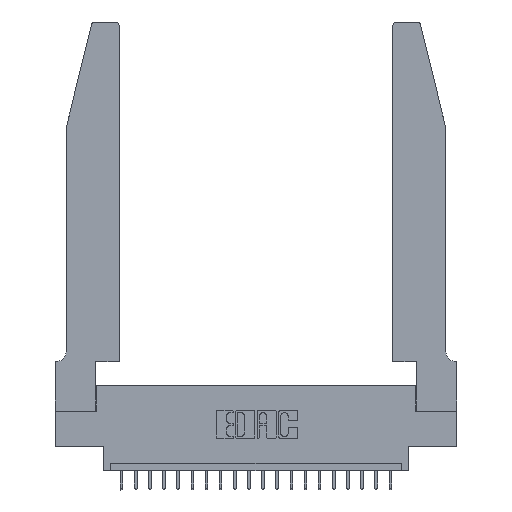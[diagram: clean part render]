
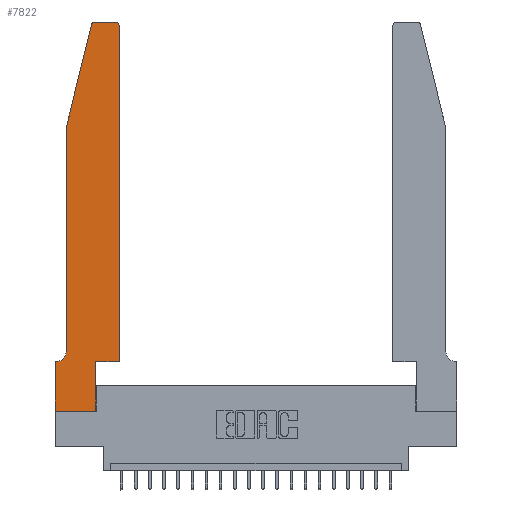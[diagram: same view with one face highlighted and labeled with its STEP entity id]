
A CAD part, top view. The second image highlights one B-rep face of the part: STEP entity #7822.
In plain terms, the highlighted planar face has unit normal (0, 0, 1).
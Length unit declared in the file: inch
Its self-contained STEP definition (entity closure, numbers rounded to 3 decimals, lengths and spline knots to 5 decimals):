
#195 = ORIENTED_EDGE ( 'NONE', *, *, #8515, .T. ) ;
#358 = CIRCLE ( 'NONE', #13378, 0.03 ) ;
#2116 = CARTESIAN_POINT ( 'NONE',  ( 0.4205, 2.72, 0.37 ) ) ;
#2129 = DIRECTION ( 'NONE',  ( 0., 0., 1. ) ) ;
#2531 = VECTOR ( 'NONE', #8893, 39.37008 ) ;
#2999 = AXIS2_PLACEMENT_3D ( 'NONE', #6093, #16201, #21540 ) ;
#3162 = CARTESIAN_POINT ( 'NONE',  ( 0.4505, 0.35, 0.37 ) ) ;
#3376 = CARTESIAN_POINT ( 'NONE',  ( 0.0755, 2., 0.37 ) ) ;
#3730 = VECTOR ( 'NONE', #6774, 39.37008 ) ;
#3759 = CARTESIAN_POINT ( 'NONE',  ( 0.284, 2.75, 0.37 ) ) ;
#3814 = EDGE_CURVE ( 'NONE', #14766, #20094, #7972, .T. ) ;
#3928 = VERTEX_POINT ( 'NONE', #4373 ) ;
#4134 = LINE ( 'NONE', #17131, #18206 ) ;
#4279 = CARTESIAN_POINT ( 'NONE',  ( 0.25487, 2.72718, 0.37 ) ) ;
#4292 = ORIENTED_EDGE ( 'NONE', *, *, #18747, .T. ) ;
#4373 = CARTESIAN_POINT ( 'NONE',  ( 0.0755, 2., 0.37 ) ) ;
#4497 = DIRECTION ( 'NONE',  ( 0., 1., 0. ) ) ;
#5254 = ORIENTED_EDGE ( 'NONE', *, *, #9867, .T. ) ;
#5349 = CARTESIAN_POINT ( 'NONE',  ( 0.2865, 0.35, 0.37 ) ) ;
#5390 = CARTESIAN_POINT ( 'NONE',  ( 0., 0., 0.37 ) ) ;
#5572 = VERTEX_POINT ( 'NONE', #3759 ) ;
#5791 = VECTOR ( 'NONE', #21121, 39.37008 ) ;
#5844 = VERTEX_POINT ( 'NONE', #10120 ) ;
#6004 = EDGE_CURVE ( 'NONE', #16092, #3928, #10452, .T. ) ;
#6049 = EDGE_CURVE ( 'NONE', #12270, #18937, #13944, .T. ) ;
#6093 = CARTESIAN_POINT ( 'NONE',  ( 0.284, 2.72, 0.37 ) ) ;
#6705 = ORIENTED_EDGE ( 'NONE', *, *, #6004, .T. ) ;
#6774 = DIRECTION ( 'NONE',  ( 1., 0., 0. ) ) ;
#6821 = VECTOR ( 'NONE', #11136, 39.37008 ) ;
#7064 = DIRECTION ( 'NONE',  ( -1., 0., 0. ) ) ;
#7257 = VECTOR ( 'NONE', #4497, 39.37008 ) ;
#7327 = VERTEX_POINT ( 'NONE', #10658 ) ;
#7358 = DIRECTION ( 'NONE',  ( 1., 0., 0. ) ) ;
#7406 = EDGE_CURVE ( 'NONE', #20196, #5572, #4134, .T. ) ;
#7476 = CARTESIAN_POINT ( 'NONE',  ( 0., 0., 0.37 ) ) ;
#7685 = DIRECTION ( 'NONE',  ( 0., 0., 1. ) ) ;
#7822 = ADVANCED_FACE ( 'NONE', ( #10844 ), #18402, .T. ) ;
#7962 = CARTESIAN_POINT ( 'NONE',  ( 0.0055, 0.35, 0.37 ) ) ;
#7972 = LINE ( 'NONE', #16586, #6821 ) ;
#8467 = ORIENTED_EDGE ( 'NONE', *, *, #7406, .T. ) ;
#8515 = EDGE_CURVE ( 'NONE', #7327, #14766, #9746, .T. ) ;
#8630 = DIRECTION ( 'NONE',  ( 1., 0., 0. ) ) ;
#8875 = CARTESIAN_POINT ( 'NONE',  ( 0., 0.35, 0.37 ) ) ;
#8893 = DIRECTION ( 'NONE',  ( 0., -1., 0. ) ) ;
#9314 = CIRCLE ( 'NONE', #2999, 0.03 ) ;
#9348 = VERTEX_POINT ( 'NONE', #11055 ) ;
#9665 = DIRECTION ( 'NONE',  ( 1., 0., 0. ) ) ;
#9746 = CIRCLE ( 'NONE', #12711, 0.07 ) ;
#9867 = EDGE_CURVE ( 'NONE', #3928, #7327, #10285, .T. ) ;
#10120 = CARTESIAN_POINT ( 'NONE',  ( 0.4505, 2.72, 0.37 ) ) ;
#10285 = LINE ( 'NONE', #17716, #2531 ) ;
#10452 = LINE ( 'NONE', #3376, #5791 ) ;
#10658 = CARTESIAN_POINT ( 'NONE',  ( 0.0755, 0.42, 0.37 ) ) ;
#10844 = FACE_OUTER_BOUND ( 'NONE', #22284, .T. ) ;
#11055 = CARTESIAN_POINT ( 'NONE',  ( 0.4505, 0.35, 0.37 ) ) ;
#11136 = DIRECTION ( 'NONE',  ( -1., 0., 0. ) ) ;
#12270 = VERTEX_POINT ( 'NONE', #15648 ) ;
#12703 = ORIENTED_EDGE ( 'NONE', *, *, #6049, .T. ) ;
#12711 = AXIS2_PLACEMENT_3D ( 'NONE', #20882, #15794, #7064 ) ;
#12807 = CARTESIAN_POINT ( 'NONE',  ( 0., 0.35, 0.37 ) ) ;
#13378 = AXIS2_PLACEMENT_3D ( 'NONE', #2116, #7685, #9665 ) ;
#13441 = LINE ( 'NONE', #20414, #7257 ) ;
#13848 = EDGE_CURVE ( 'NONE', #5572, #16092, #9314, .T. ) ;
#13944 = LINE ( 'NONE', #5349, #20595 ) ;
#14553 = DIRECTION ( 'NONE',  ( 0., -1., 0. ) ) ;
#14766 = VERTEX_POINT ( 'NONE', #7962 ) ;
#14827 = LINE ( 'NONE', #3162, #3730 ) ;
#14840 = ORIENTED_EDGE ( 'NONE', *, *, #16865, .T. ) ;
#15648 = CARTESIAN_POINT ( 'NONE',  ( 0.2865, 0., 0.37 ) ) ;
#15794 = DIRECTION ( 'NONE',  ( 0., 0., -1. ) ) ;
#16092 = VERTEX_POINT ( 'NONE', #4279 ) ;
#16113 = EDGE_CURVE ( 'NONE', #9348, #5844, #13441, .T. ) ;
#16201 = DIRECTION ( 'NONE',  ( 0., 0., 1. ) ) ;
#16486 = EDGE_CURVE ( 'NONE', #18937, #9348, #14827, .T. ) ;
#16521 = VECTOR ( 'NONE', #14553, 39.37008 ) ;
#16586 = CARTESIAN_POINT ( 'NONE',  ( 0.0755, 0.35, 0.37 ) ) ;
#16780 = AXIS2_PLACEMENT_3D ( 'NONE', #12807, #2129, #7358 ) ;
#16865 = EDGE_CURVE ( 'NONE', #5844, #20196, #358, .T. ) ;
#16872 = CARTESIAN_POINT ( 'NONE',  ( 0.2865, 0.35, 0.37 ) ) ;
#16915 = ORIENTED_EDGE ( 'NONE', *, *, #16486, .T. ) ;
#17131 = CARTESIAN_POINT ( 'NONE',  ( 0.2605, 2.75, 0.37 ) ) ;
#17239 = ORIENTED_EDGE ( 'NONE', *, *, #3814, .T. ) ;
#17716 = CARTESIAN_POINT ( 'NONE',  ( 0.0755, 2., 0.37 ) ) ;
#17751 = EDGE_CURVE ( 'NONE', #20823, #12270, #17817, .T. ) ;
#17814 = LINE ( 'NONE', #7476, #16521 ) ;
#17817 = LINE ( 'NONE', #5390, #18736 ) ;
#18206 = VECTOR ( 'NONE', #18853, 39.37008 ) ;
#18288 = ORIENTED_EDGE ( 'NONE', *, *, #17751, .T. ) ;
#18402 = PLANE ( 'NONE',  #16780 ) ;
#18736 = VECTOR ( 'NONE', #8630, 39.37008 ) ;
#18747 = EDGE_CURVE ( 'NONE', #20094, #20823, #17814, .T. ) ;
#18853 = DIRECTION ( 'NONE',  ( -1., 0., 0. ) ) ;
#18937 = VERTEX_POINT ( 'NONE', #16872 ) ;
#19512 = DIRECTION ( 'NONE',  ( 0., 1., 0. ) ) ;
#20094 = VERTEX_POINT ( 'NONE', #8875 ) ;
#20196 = VERTEX_POINT ( 'NONE', #21984 ) ;
#20414 = CARTESIAN_POINT ( 'NONE',  ( 0.4505, 0.35, 0.37 ) ) ;
#20595 = VECTOR ( 'NONE', #19512, 39.37008 ) ;
#20669 = CARTESIAN_POINT ( 'NONE',  ( 0., 0., 0.37 ) ) ;
#20823 = VERTEX_POINT ( 'NONE', #20669 ) ;
#20879 = ORIENTED_EDGE ( 'NONE', *, *, #13848, .T. ) ;
#20882 = CARTESIAN_POINT ( 'NONE',  ( 0.0055, 0.42, 0.37 ) ) ;
#21121 = DIRECTION ( 'NONE',  ( -0.239, -0.971, 0. ) ) ;
#21540 = DIRECTION ( 'NONE',  ( 1., 0., 0. ) ) ;
#21613 = ORIENTED_EDGE ( 'NONE', *, *, #16113, .T. ) ;
#21984 = CARTESIAN_POINT ( 'NONE',  ( 0.4205, 2.75, 0.37 ) ) ;
#22284 = EDGE_LOOP ( 'NONE', ( #8467, #20879, #6705, #5254, #195, #17239, #4292, #18288, #12703, #16915, #21613, #14840 ) ) ;
